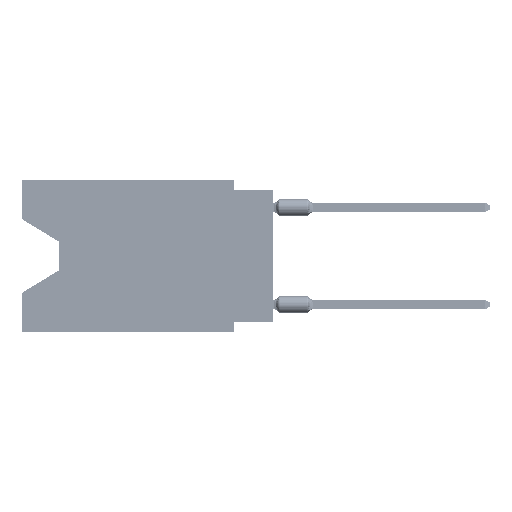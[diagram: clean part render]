
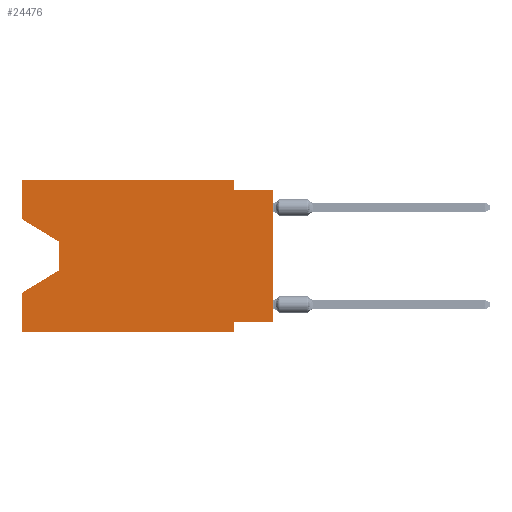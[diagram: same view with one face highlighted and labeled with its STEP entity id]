
A CAD part, left-side view. The second image highlights one B-rep face of the part: STEP entity #24476.
In plain terms, the highlighted planar face has unit normal (-1, 0, 0).
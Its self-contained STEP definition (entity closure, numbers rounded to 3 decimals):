
#705 = EDGE_CURVE ( 'NONE', #31213, #34418, #21289, .T. ) ;
#974 = EDGE_CURVE ( 'NONE', #13387, #59366, #31774, .T. ) ;
#1394 = CARTESIAN_POINT ( 'NONE',  ( 0., 16.383, 0. ) ) ;
#1817 = EDGE_CURVE ( 'NONE', #59366, #16835, #17798, .T. ) ;
#2187 = LINE ( 'NONE', #1394, #61026 ) ;
#4019 = CARTESIAN_POINT ( 'NONE',  ( 0., 16.383, 0. ) ) ;
#4352 = EDGE_CURVE ( 'NONE', #26943, #13387, #52416, .T. ) ;
#4617 = EDGE_CURVE ( 'NONE', #68822, #67173, #64819, .T. ) ;
#6448 = VERTEX_POINT ( 'NONE', #59132 ) ;
#9067 = VERTEX_POINT ( 'NONE', #72216 ) ;
#9793 = EDGE_CURVE ( 'NONE', #40972, #9067, #36186, .T. ) ;
#11703 = ORIENTED_EDGE ( 'NONE', *, *, #705, .F. ) ;
#11810 = DIRECTION ( 'NONE',  ( 0., 0., -1. ) ) ;
#12210 = VECTOR ( 'NONE', #78404, 1000. ) ;
#12500 = CARTESIAN_POINT ( 'NONE',  ( 0., 13.97, -5.893 ) ) ;
#13387 = VERTEX_POINT ( 'NONE', #79795 ) ;
#13681 = PLANE ( 'NONE',  #47247 ) ;
#13839 = DIRECTION ( 'NONE',  ( 0., 0., -1. ) ) ;
#15383 = DIRECTION ( 'NONE',  ( 0., 1., 0. ) ) ;
#15870 = CARTESIAN_POINT ( 'NONE',  ( 0., 16.383, -2.546 ) ) ;
#16611 = VECTOR ( 'NONE', #41549, 1000. ) ;
#16835 = VERTEX_POINT ( 'NONE', #37278 ) ;
#17692 = LINE ( 'NONE', #59532, #23645 ) ;
#17798 = LINE ( 'NONE', #12500, #19870 ) ;
#18940 = CARTESIAN_POINT ( 'NONE',  ( 0., 0., -0.635 ) ) ;
#19870 = VECTOR ( 'NONE', #62036, 1000. ) ;
#21289 = LINE ( 'NONE', #27767, #48213 ) ;
#22594 = VECTOR ( 'NONE', #13839, 1000. ) ;
#22887 = CARTESIAN_POINT ( 'NONE',  ( 0., 16.383, 0. ) ) ;
#23064 = EDGE_CURVE ( 'NONE', #6448, #67173, #72671, .T. ) ;
#23604 = ORIENTED_EDGE ( 'NONE', *, *, #49724, .F. ) ;
#23645 = VECTOR ( 'NONE', #47752, 1000. ) ;
#24081 = ORIENTED_EDGE ( 'NONE', *, *, #54480, .F. ) ;
#24476 = ADVANCED_FACE ( 'NONE', ( #44535 ), #13681, .F. ) ;
#26603 = ORIENTED_EDGE ( 'NONE', *, *, #4352, .T. ) ;
#26671 = CARTESIAN_POINT ( 'NONE',  ( 0., 16.383, 0. ) ) ;
#26943 = VERTEX_POINT ( 'NONE', #45371 ) ;
#27767 = CARTESIAN_POINT ( 'NONE',  ( 0., 16.383, 0. ) ) ;
#27943 = EDGE_CURVE ( 'NONE', #49595, #16835, #2187, .T. ) ;
#30337 = EDGE_CURVE ( 'NONE', #49595, #9067, #17692, .T. ) ;
#30976 = CARTESIAN_POINT ( 'NONE',  ( 0., 13.97, -4.013 ) ) ;
#31213 = VERTEX_POINT ( 'NONE', #4019 ) ;
#31536 = CARTESIAN_POINT ( 'NONE',  ( 0., 0., -9.271 ) ) ;
#31658 = DIRECTION ( 'NONE',  ( 0., 0., 1. ) ) ;
#31774 = LINE ( 'NONE', #30976, #43043 ) ;
#32903 = ORIENTED_EDGE ( 'NONE', *, *, #4617, .T. ) ;
#33998 = ORIENTED_EDGE ( 'NONE', *, *, #974, .T. ) ;
#34418 = VERTEX_POINT ( 'NONE', #59617 ) ;
#34818 = ORIENTED_EDGE ( 'NONE', *, *, #1817, .T. ) ;
#36186 = LINE ( 'NONE', #41856, #51709 ) ;
#37033 = VECTOR ( 'NONE', #15383, 1000. ) ;
#37220 = ORIENTED_EDGE ( 'NONE', *, *, #67020, .F. ) ;
#37278 = CARTESIAN_POINT ( 'NONE',  ( 0., 16.383, -7.36 ) ) ;
#40731 = VECTOR ( 'NONE', #31658, 1000. ) ;
#40972 = VERTEX_POINT ( 'NONE', #67685 ) ;
#41005 = CARTESIAN_POINT ( 'NONE',  ( 0., 0., -0.635 ) ) ;
#41549 = DIRECTION ( 'NONE',  ( 0., 0., 1. ) ) ;
#41856 = CARTESIAN_POINT ( 'NONE',  ( 0., 2.54, -9.906 ) ) ;
#43043 = VECTOR ( 'NONE', #55731, 1000. ) ;
#44535 = FACE_OUTER_BOUND ( 'NONE', #59460, .T. ) ;
#44695 = LINE ( 'NONE', #69461, #22594 ) ;
#45371 = CARTESIAN_POINT ( 'NONE',  ( 0., 16.383, -2.546 ) ) ;
#47247 = AXIS2_PLACEMENT_3D ( 'NONE', #26671, #69304, #51431 ) ;
#47752 = DIRECTION ( 'NONE',  ( 0., -1., 0. ) ) ;
#47771 = ORIENTED_EDGE ( 'NONE', *, *, #23064, .F. ) ;
#48213 = VECTOR ( 'NONE', #77326, 1000. ) ;
#49595 = VERTEX_POINT ( 'NONE', #79093 ) ;
#49724 = EDGE_CURVE ( 'NONE', #26943, #31213, #79298, .T. ) ;
#51431 = DIRECTION ( 'NONE',  ( 0., 0., -1. ) ) ;
#51709 = VECTOR ( 'NONE', #11810, 1000. ) ;
#52327 = CARTESIAN_POINT ( 'NONE',  ( 0., 0., -9.271 ) ) ;
#52416 = LINE ( 'NONE', #15870, #12210 ) ;
#53653 = ORIENTED_EDGE ( 'NONE', *, *, #9793, .F. ) ;
#54480 = EDGE_CURVE ( 'NONE', #68822, #40972, #77916, .T. ) ;
#55731 = DIRECTION ( 'NONE',  ( 0., 0., -1. ) ) ;
#56009 = CARTESIAN_POINT ( 'NONE',  ( 0., 0., 0. ) ) ;
#59132 = CARTESIAN_POINT ( 'NONE',  ( 0., 2.54, -0.635 ) ) ;
#59366 = VERTEX_POINT ( 'NONE', #78562 ) ;
#59460 = EDGE_LOOP ( 'NONE', ( #26603, #33998, #34818, #64627, #79959, #53653, #24081, #32903, #47771, #37220, #11703, #23604 ) ) ;
#59532 = CARTESIAN_POINT ( 'NONE',  ( 0., 16.383, -9.906 ) ) ;
#59617 = CARTESIAN_POINT ( 'NONE',  ( 0., 2.54, 0. ) ) ;
#61026 = VECTOR ( 'NONE', #62692, 1000. ) ;
#62036 = DIRECTION ( 'NONE',  ( 0., 0.855, -0.519 ) ) ;
#62692 = DIRECTION ( 'NONE',  ( 0., 0., 1. ) ) ;
#64627 = ORIENTED_EDGE ( 'NONE', *, *, #27943, .F. ) ;
#64819 = LINE ( 'NONE', #56009, #40731 ) ;
#66175 = DIRECTION ( 'NONE',  ( 0., -1., 0. ) ) ;
#67020 = EDGE_CURVE ( 'NONE', #34418, #6448, #44695, .T. ) ;
#67173 = VERTEX_POINT ( 'NONE', #18940 ) ;
#67685 = CARTESIAN_POINT ( 'NONE',  ( 0., 2.54, -9.271 ) ) ;
#68822 = VERTEX_POINT ( 'NONE', #31536 ) ;
#69304 = DIRECTION ( 'NONE',  ( 1., 0., 0. ) ) ;
#69461 = CARTESIAN_POINT ( 'NONE',  ( 0., 2.54, 0. ) ) ;
#72216 = CARTESIAN_POINT ( 'NONE',  ( 0., 2.54, -9.906 ) ) ;
#72671 = LINE ( 'NONE', #41005, #75658 ) ;
#75658 = VECTOR ( 'NONE', #66175, 1000. ) ;
#77326 = DIRECTION ( 'NONE',  ( 0., -1., 0. ) ) ;
#77916 = LINE ( 'NONE', #52327, #37033 ) ;
#78404 = DIRECTION ( 'NONE',  ( 0., -0.855, -0.519 ) ) ;
#78562 = CARTESIAN_POINT ( 'NONE',  ( 0., 13.97, -5.893 ) ) ;
#79093 = CARTESIAN_POINT ( 'NONE',  ( 0., 16.383, -9.906 ) ) ;
#79298 = LINE ( 'NONE', #22887, #16611 ) ;
#79795 = CARTESIAN_POINT ( 'NONE',  ( 0., 13.97, -4.013 ) ) ;
#79959 = ORIENTED_EDGE ( 'NONE', *, *, #30337, .T. ) ;
